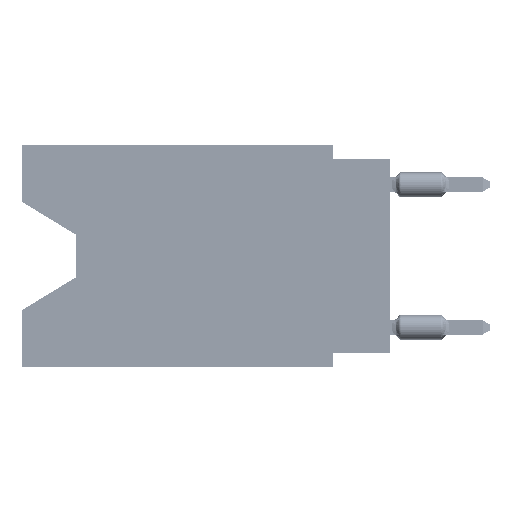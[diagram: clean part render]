
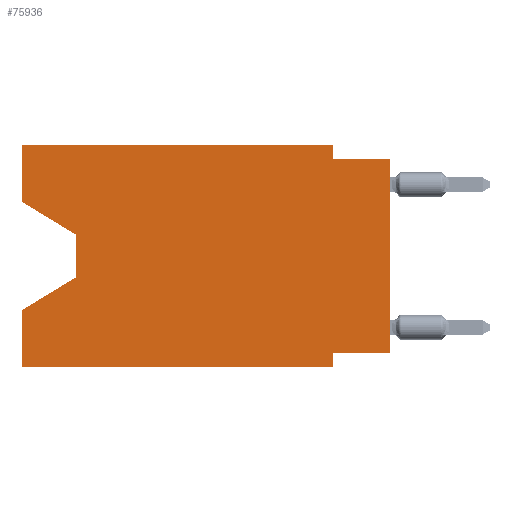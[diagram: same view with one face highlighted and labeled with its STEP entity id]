
A CAD part, left-side view. The second image highlights one B-rep face of the part: STEP entity #75936.
In plain terms, the highlighted planar face has unit normal (-1, 0, 0).
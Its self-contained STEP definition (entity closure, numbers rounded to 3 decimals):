
#626 = DIRECTION ( 'NONE',  ( 0., 0.855, -0.519 ) ) ;
#1165 = LINE ( 'NONE', #17398, #38444 ) ;
#1935 = EDGE_CURVE ( 'NONE', #73549, #71311, #3165, .T. ) ;
#1937 = VECTOR ( 'NONE', #3541, 1000. ) ;
#2318 = ORIENTED_EDGE ( 'NONE', *, *, #60437, .T. ) ;
#2339 = AXIS2_PLACEMENT_3D ( 'NONE', #29128, #27973, #23326 ) ;
#3086 = EDGE_CURVE ( 'NONE', #25321, #34601, #49920, .T. ) ;
#3165 = LINE ( 'NONE', #62173, #1937 ) ;
#3541 = DIRECTION ( 'NONE',  ( 0., 1., 0. ) ) ;
#4304 = EDGE_CURVE ( 'NONE', #48322, #34241, #67262, .T. ) ;
#5773 = LINE ( 'NONE', #52838, #65206 ) ;
#5898 = DIRECTION ( 'NONE',  ( 0., 0., -1. ) ) ;
#6800 = CARTESIAN_POINT ( 'NONE',  ( 0., 13.97, -5.893 ) ) ;
#7555 = LINE ( 'NONE', #6800, #37625 ) ;
#7897 = DIRECTION ( 'NONE',  ( 0., -0.855, -0.519 ) ) ;
#10451 = DIRECTION ( 'NONE',  ( 0., -1., 0. ) ) ;
#10710 = CARTESIAN_POINT ( 'NONE',  ( 0., 13.97, -4.013 ) ) ;
#14014 = EDGE_CURVE ( 'NONE', #55289, #26545, #22025, .T. ) ;
#14075 = CARTESIAN_POINT ( 'NONE',  ( 0., 16.383, 0. ) ) ;
#17026 = EDGE_CURVE ( 'NONE', #71311, #39446, #53729, .T. ) ;
#17398 = CARTESIAN_POINT ( 'NONE',  ( 0., 2.54, 0. ) ) ;
#18264 = ORIENTED_EDGE ( 'NONE', *, *, #22463, .T. ) ;
#18508 = DIRECTION ( 'NONE',  ( 0., 0., 1. ) ) ;
#18920 = CARTESIAN_POINT ( 'NONE',  ( 0., 16.383, -2.546 ) ) ;
#18929 = VECTOR ( 'NONE', #10451, 1000. ) ;
#19921 = LINE ( 'NONE', #62676, #58048 ) ;
#19923 = ORIENTED_EDGE ( 'NONE', *, *, #1935, .F. ) ;
#20512 = VECTOR ( 'NONE', #7897, 1000. ) ;
#21402 = ORIENTED_EDGE ( 'NONE', *, *, #58568, .F. ) ;
#22025 = LINE ( 'NONE', #57127, #18929 ) ;
#22463 = EDGE_CURVE ( 'NONE', #73549, #26545, #61296, .T. ) ;
#22844 = ORIENTED_EDGE ( 'NONE', *, *, #17026, .F. ) ;
#23326 = DIRECTION ( 'NONE',  ( 0., 0., -1. ) ) ;
#24098 = ORIENTED_EDGE ( 'NONE', *, *, #44243, .F. ) ;
#24656 = CARTESIAN_POINT ( 'NONE',  ( 0., 2.54, -0.635 ) ) ;
#24715 = LINE ( 'NONE', #25094, #52135 ) ;
#25094 = CARTESIAN_POINT ( 'NONE',  ( 0., 13.97, -4.013 ) ) ;
#25321 = VERTEX_POINT ( 'NONE', #55984 ) ;
#25843 = EDGE_LOOP ( 'NONE', ( #44728, #59092, #28337, #60782, #2318, #22844, #19923, #18264, #37345, #24098, #70477, #21402 ) ) ;
#25868 = DIRECTION ( 'NONE',  ( 0., -1., 0. ) ) ;
#26545 = VERTEX_POINT ( 'NONE', #53282 ) ;
#27973 = DIRECTION ( 'NONE',  ( 1., 0., 0. ) ) ;
#28337 = ORIENTED_EDGE ( 'NONE', *, *, #52847, .T. ) ;
#29068 = CARTESIAN_POINT ( 'NONE',  ( 0., 2.54, -9.906 ) ) ;
#29128 = CARTESIAN_POINT ( 'NONE',  ( 0., 16.383, 0. ) ) ;
#29499 = CARTESIAN_POINT ( 'NONE',  ( 0., 13.97, -5.893 ) ) ;
#30049 = CARTESIAN_POINT ( 'NONE',  ( 0., 2.54, -9.906 ) ) ;
#31501 = DIRECTION ( 'NONE',  ( 0., -1., 0. ) ) ;
#31802 = DIRECTION ( 'NONE',  ( 0., 0., 1. ) ) ;
#33749 = PLANE ( 'NONE',  #2339 ) ;
#34241 = VERTEX_POINT ( 'NONE', #10710 ) ;
#34519 = FACE_OUTER_BOUND ( 'NONE', #25843, .T. ) ;
#34601 = VERTEX_POINT ( 'NONE', #42328 ) ;
#37229 = CARTESIAN_POINT ( 'NONE',  ( 0., 16.383, -2.546 ) ) ;
#37345 = ORIENTED_EDGE ( 'NONE', *, *, #14014, .F. ) ;
#37428 = CARTESIAN_POINT ( 'NONE',  ( 0., 0., 0. ) ) ;
#37625 = VECTOR ( 'NONE', #626, 1000. ) ;
#37737 = CARTESIAN_POINT ( 'NONE',  ( 0., 16.383, 0. ) ) ;
#38444 = VECTOR ( 'NONE', #40929, 1000. ) ;
#39446 = VERTEX_POINT ( 'NONE', #30049 ) ;
#40929 = DIRECTION ( 'NONE',  ( 0., 0., -1. ) ) ;
#42328 = CARTESIAN_POINT ( 'NONE',  ( 0., 16.383, -7.36 ) ) ;
#42836 = DIRECTION ( 'NONE',  ( 0., 0., -1. ) ) ;
#43776 = CARTESIAN_POINT ( 'NONE',  ( 0., 2.54, -9.271 ) ) ;
#44000 = VECTOR ( 'NONE', #55909, 1000. ) ;
#44243 = EDGE_CURVE ( 'NONE', #46081, #55289, #1165, .T. ) ;
#44728 = ORIENTED_EDGE ( 'NONE', *, *, #4304, .T. ) ;
#46081 = VERTEX_POINT ( 'NONE', #76131 ) ;
#46312 = VECTOR ( 'NONE', #25868, 1000. ) ;
#47194 = VERTEX_POINT ( 'NONE', #29499 ) ;
#48322 = VERTEX_POINT ( 'NONE', #18920 ) ;
#49920 = LINE ( 'NONE', #14075, #62376 ) ;
#52135 = VECTOR ( 'NONE', #42836, 1000. ) ;
#52838 = CARTESIAN_POINT ( 'NONE',  ( 0., 16.383, 0. ) ) ;
#52847 = EDGE_CURVE ( 'NONE', #47194, #34601, #7555, .T. ) ;
#53282 = CARTESIAN_POINT ( 'NONE',  ( 0., 0., -0.635 ) ) ;
#53729 = LINE ( 'NONE', #29068, #60913 ) ;
#53770 = EDGE_CURVE ( 'NONE', #73572, #46081, #58691, .T. ) ;
#55289 = VERTEX_POINT ( 'NONE', #24656 ) ;
#55909 = DIRECTION ( 'NONE',  ( 0., 0., 1. ) ) ;
#55984 = CARTESIAN_POINT ( 'NONE',  ( 0., 16.383, -9.906 ) ) ;
#57127 = CARTESIAN_POINT ( 'NONE',  ( 0., 0., -0.635 ) ) ;
#58048 = VECTOR ( 'NONE', #31501, 1000. ) ;
#58568 = EDGE_CURVE ( 'NONE', #48322, #73572, #5773, .T. ) ;
#58691 = LINE ( 'NONE', #70650, #46312 ) ;
#59092 = ORIENTED_EDGE ( 'NONE', *, *, #71722, .T. ) ;
#60437 = EDGE_CURVE ( 'NONE', #25321, #39446, #19921, .T. ) ;
#60782 = ORIENTED_EDGE ( 'NONE', *, *, #3086, .F. ) ;
#60913 = VECTOR ( 'NONE', #5898, 1000. ) ;
#61296 = LINE ( 'NONE', #37428, #44000 ) ;
#62173 = CARTESIAN_POINT ( 'NONE',  ( 0., 0., -9.271 ) ) ;
#62376 = VECTOR ( 'NONE', #31802, 1000. ) ;
#62676 = CARTESIAN_POINT ( 'NONE',  ( 0., 16.383, -9.906 ) ) ;
#65206 = VECTOR ( 'NONE', #18508, 1000. ) ;
#67262 = LINE ( 'NONE', #37229, #20512 ) ;
#68151 = CARTESIAN_POINT ( 'NONE',  ( 0., 0., -9.271 ) ) ;
#70477 = ORIENTED_EDGE ( 'NONE', *, *, #53770, .F. ) ;
#70650 = CARTESIAN_POINT ( 'NONE',  ( 0., 16.383, 0. ) ) ;
#71311 = VERTEX_POINT ( 'NONE', #43776 ) ;
#71722 = EDGE_CURVE ( 'NONE', #34241, #47194, #24715, .T. ) ;
#73549 = VERTEX_POINT ( 'NONE', #68151 ) ;
#73572 = VERTEX_POINT ( 'NONE', #37737 ) ;
#75936 = ADVANCED_FACE ( 'NONE', ( #34519 ), #33749, .F. ) ;
#76131 = CARTESIAN_POINT ( 'NONE',  ( 0., 2.54, 0. ) ) ;
